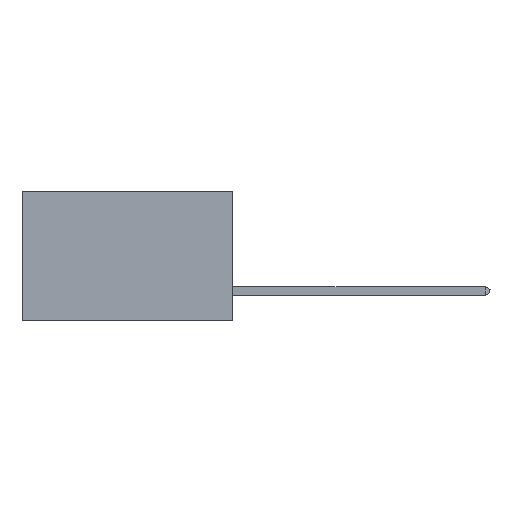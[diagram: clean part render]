
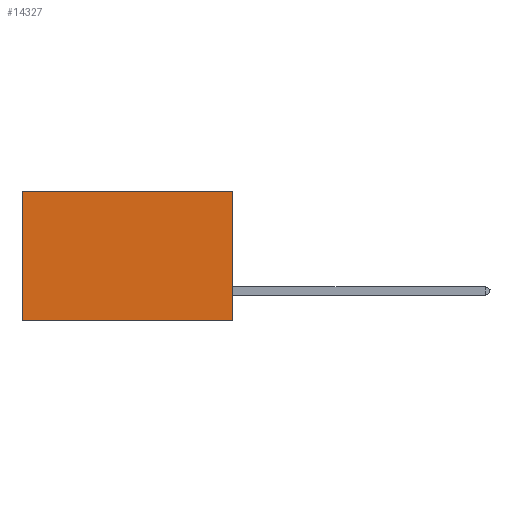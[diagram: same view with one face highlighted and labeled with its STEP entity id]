
A CAD part, left-side view. The second image highlights one B-rep face of the part: STEP entity #14327.
In plain terms, the highlighted planar face has unit normal (-1, 0, 0).
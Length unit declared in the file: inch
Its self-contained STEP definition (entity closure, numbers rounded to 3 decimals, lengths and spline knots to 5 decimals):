
#1721 = AXIS2_PLACEMENT_3D ( 'NONE', #11893, #8769, #12040 ) ;
#1987 = CARTESIAN_POINT ( 'NONE',  ( 0.2875, 0., 0. ) ) ;
#2930 = FACE_OUTER_BOUND ( 'NONE', #31642, .T. ) ;
#4146 = EDGE_CURVE ( 'NONE', #29201, #17512, #33672, .T. ) ;
#5494 = ORIENTED_EDGE ( 'NONE', *, *, #38273, .F. ) ;
#7522 = DIRECTION ( 'NONE',  ( 0., 0., -1. ) ) ;
#7897 = DIRECTION ( 'NONE',  ( 0., 0., -1. ) ) ;
#8296 = CARTESIAN_POINT ( 'NONE',  ( 0.2875, 0., 0. ) ) ;
#8769 = DIRECTION ( 'NONE',  ( 1., 0., 0. ) ) ;
#11340 = ORIENTED_EDGE ( 'NONE', *, *, #30869, .T. ) ;
#11475 = VECTOR ( 'NONE', #7522, 39.37008 ) ;
#11893 = CARTESIAN_POINT ( 'NONE',  ( 0.2875, 0., 0. ) ) ;
#11947 = LINE ( 'NONE', #36737, #11475 ) ;
#12040 = DIRECTION ( 'NONE',  ( 0., 0., -1. ) ) ;
#13834 = VECTOR ( 'NONE', #22973, 39.37008 ) ;
#14243 = VERTEX_POINT ( 'NONE', #1987 ) ;
#14327 = ADVANCED_FACE ( 'NONE', ( #2930 ), #41064, .F. ) ;
#16411 = DIRECTION ( 'NONE',  ( 0., 1., 0. ) ) ;
#16784 = VERTEX_POINT ( 'NONE', #37222 ) ;
#17512 = VERTEX_POINT ( 'NONE', #19016 ) ;
#19016 = CARTESIAN_POINT ( 'NONE',  ( 0.2875, 0.6, -0.37 ) ) ;
#19751 = LINE ( 'NONE', #8296, #26369 ) ;
#22832 = CARTESIAN_POINT ( 'NONE',  ( 0.2875, 0., 0. ) ) ;
#22973 = DIRECTION ( 'NONE',  ( 0., 1., 0. ) ) ;
#26369 = VECTOR ( 'NONE', #7897, 39.37008 ) ;
#29201 = VERTEX_POINT ( 'NONE', #33628 ) ;
#30869 = EDGE_CURVE ( 'NONE', #14243, #16784, #37116, .T. ) ;
#31642 = EDGE_LOOP ( 'NONE', ( #41970, #33779, #5494, #11340 ) ) ;
#33045 = CARTESIAN_POINT ( 'NONE',  ( 0.2875, 0., -0.37 ) ) ;
#33572 = EDGE_CURVE ( 'NONE', #16784, #17512, #11947, .T. ) ;
#33628 = CARTESIAN_POINT ( 'NONE',  ( 0.2875, 0., -0.37 ) ) ;
#33672 = LINE ( 'NONE', #33045, #13834 ) ;
#33779 = ORIENTED_EDGE ( 'NONE', *, *, #4146, .F. ) ;
#36042 = VECTOR ( 'NONE', #16411, 39.37008 ) ;
#36737 = CARTESIAN_POINT ( 'NONE',  ( 0.2875, 0.6, 0. ) ) ;
#37116 = LINE ( 'NONE', #22832, #36042 ) ;
#37222 = CARTESIAN_POINT ( 'NONE',  ( 0.2875, 0.6, 0. ) ) ;
#38273 = EDGE_CURVE ( 'NONE', #14243, #29201, #19751, .T. ) ;
#41064 = PLANE ( 'NONE',  #1721 ) ;
#41970 = ORIENTED_EDGE ( 'NONE', *, *, #33572, .T. ) ;
